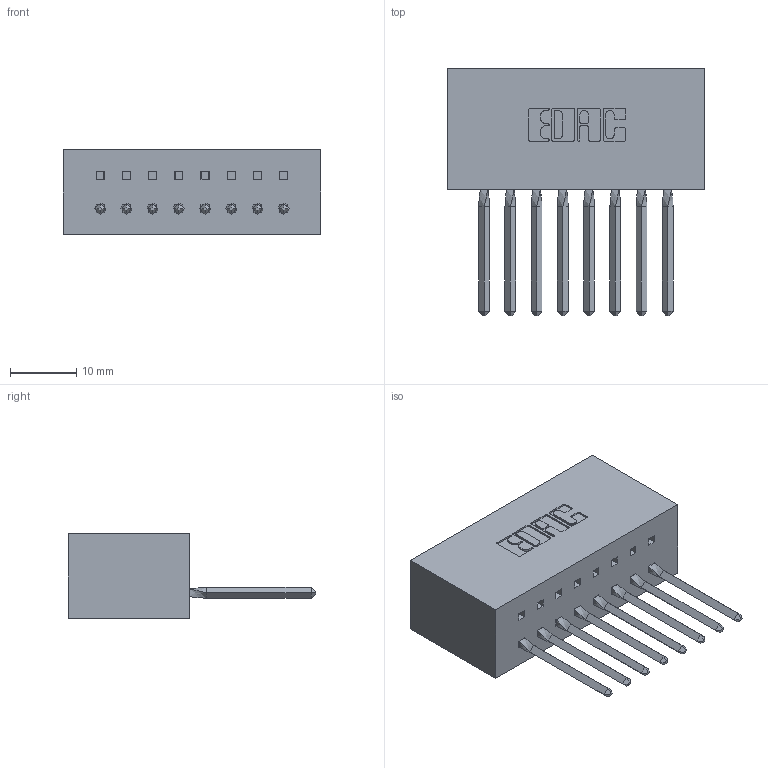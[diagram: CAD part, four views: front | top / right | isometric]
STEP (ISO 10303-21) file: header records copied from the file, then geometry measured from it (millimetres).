
FILE_DESCRIPTION (( 'STEP AP203' ), '1' );
FILE_NAME ('317-008-541-601.STEP', '2020-02-27T13:07:16', ( '' ), ( '' ), 'SwSTEP 2.0', 'SolidWorks 2016', '' );
FILE_SCHEMA (( 'CONFIG_CONTROL_DESIGN' ));
Length unit declared in the file: inch
Products named in the file (3): 317-008-541-601; 317-290-002_541; 317 Part_Lugless
Assembly tree (9 placements, depth 2):
  317-008-541-601
    317 Part_Lugless
    317-290-002_541  x8
Bounding box: 38.91 x 37.34 x 12.7 mm (x, y, z)
Volume: 6970.7 mm3; surface area: 8910.2 mm2
Topology: 9 solids, 9 shells, 1306 faces, 3711 edges, 2414 vertices
Faces by surface type: plane 1042, cylinder 232, bspline 32
Entity records: 17190 total; most frequent: CARTESIAN_POINT 3681, ORIENTED_EDGE 2942, DIRECTION 2383, EDGE_CURVE 1471, VECTOR 1115, LINE 1115, VERTEX_POINT 972, AXIS2_PLACEMENT_3D 634
